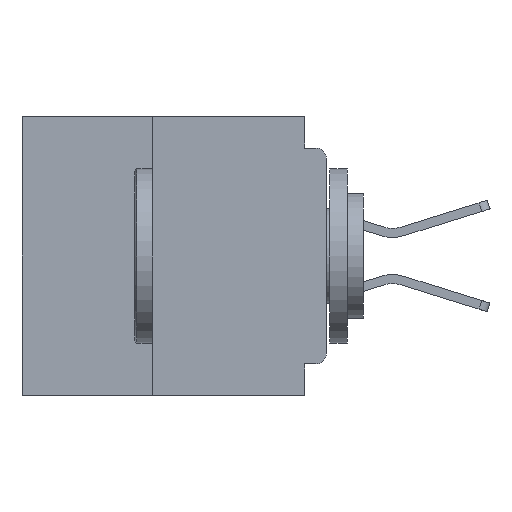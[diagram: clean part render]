
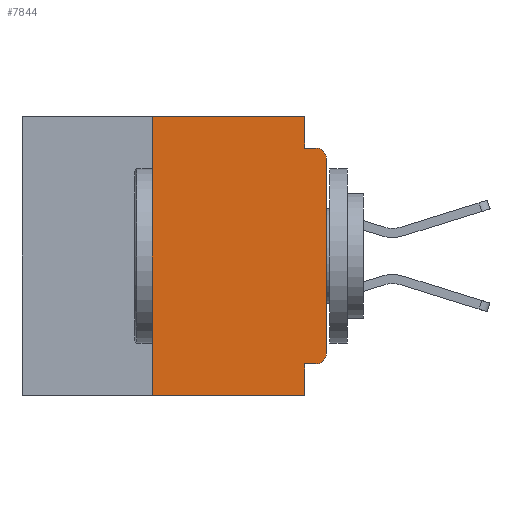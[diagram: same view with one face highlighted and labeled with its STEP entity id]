
A CAD part, left-side view. The second image highlights one B-rep face of the part: STEP entity #7844.
In plain terms, the highlighted planar face has unit normal (-1, 0, 0).
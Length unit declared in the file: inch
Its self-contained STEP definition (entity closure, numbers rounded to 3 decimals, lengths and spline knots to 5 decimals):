
#17 = EDGE_CURVE ( 'NONE', #37100, #36242, #29036, .T. ) ;
#1278 = DIRECTION ( 'NONE',  ( -1., 0., 0. ) ) ;
#3343 = CARTESIAN_POINT ( 'NONE',  ( 0., 0., -0.34 ) ) ;
#3614 = CARTESIAN_POINT ( 'NONE',  ( 0., 0.031, 0. ) ) ;
#3674 = LINE ( 'NONE', #17124, #46001 ) ;
#4310 = DIRECTION ( 'NONE',  ( -1., 0., 0. ) ) ;
#5064 = VECTOR ( 'NONE', #15952, 39.37008 ) ;
#5339 = CARTESIAN_POINT ( 'NONE',  ( 0., 0.25, -0.4 ) ) ;
#6149 = VERTEX_POINT ( 'NONE', #40076 ) ;
#6697 = PLANE ( 'NONE',  #9297 ) ;
#6918 = VECTOR ( 'NONE', #46391, 39.37008 ) ;
#7844 = ADVANCED_FACE ( 'NONE', ( #22489 ), #6697, .F. ) ;
#8098 = CIRCLE ( 'NONE', #25250, 0.015 ) ;
#9297 = AXIS2_PLACEMENT_3D ( 'NONE', #43621, #19162, #47717 ) ;
#9511 = LINE ( 'NONE', #15062, #20519 ) ;
#9533 = EDGE_CURVE ( 'NONE', #40594, #33171, #8098, .T. ) ;
#11437 = EDGE_CURVE ( 'NONE', #38877, #35262, #44872, .T. ) ;
#13422 = DIRECTION ( 'NONE',  ( 0., -1., 0. ) ) ;
#13489 = CARTESIAN_POINT ( 'NONE',  ( 0., 0.25, -0.4 ) ) ;
#13791 = VERTEX_POINT ( 'NONE', #50449 ) ;
#15062 = CARTESIAN_POINT ( 'NONE',  ( 0., 0., -0.355 ) ) ;
#15172 = VERTEX_POINT ( 'NONE', #24614 ) ;
#15555 = ORIENTED_EDGE ( 'NONE', *, *, #27257, .F. ) ;
#15952 = DIRECTION ( 'NONE',  ( 0., -1., 0. ) ) ;
#15962 = DIRECTION ( 'NONE',  ( 0., -1., 0. ) ) ;
#17124 = CARTESIAN_POINT ( 'NONE',  ( 0., 0.031, -0.4 ) ) ;
#17565 = CARTESIAN_POINT ( 'NONE',  ( 0., 0.437, -0.4 ) ) ;
#18684 = ORIENTED_EDGE ( 'NONE', *, *, #9533, .T. ) ;
#19162 = DIRECTION ( 'NONE',  ( 1., 0., 0. ) ) ;
#19197 = DIRECTION ( 'NONE',  ( 0., 1., 0. ) ) ;
#20519 = VECTOR ( 'NONE', #19197, 39.37008 ) ;
#21345 = AXIS2_PLACEMENT_3D ( 'NONE', #29032, #4310, #33144 ) ;
#21432 = CARTESIAN_POINT ( 'NONE',  ( 0., 0.015, -0.355 ) ) ;
#21860 = EDGE_CURVE ( 'NONE', #40594, #6149, #9511, .T. ) ;
#21900 = LINE ( 'NONE', #48632, #23185 ) ;
#22489 = FACE_OUTER_BOUND ( 'NONE', #43771, .T. ) ;
#23185 = VECTOR ( 'NONE', #15962, 39.37008 ) ;
#24335 = DIRECTION ( 'NONE',  ( 0., 0., -1. ) ) ;
#24614 = CARTESIAN_POINT ( 'NONE',  ( 0., 0., -0.06 ) ) ;
#25250 = AXIS2_PLACEMENT_3D ( 'NONE', #26008, #1278, #30164 ) ;
#26008 = CARTESIAN_POINT ( 'NONE',  ( 0., 0.015, -0.34 ) ) ;
#26440 = ORIENTED_EDGE ( 'NONE', *, *, #46007, .F. ) ;
#27059 = ORIENTED_EDGE ( 'NONE', *, *, #40671, .F. ) ;
#27257 = EDGE_CURVE ( 'NONE', #36242, #51646, #21900, .T. ) ;
#28770 = ORIENTED_EDGE ( 'NONE', *, *, #11437, .T. ) ;
#29032 = CARTESIAN_POINT ( 'NONE',  ( 0., 0.015, -0.06 ) ) ;
#29036 = LINE ( 'NONE', #3614, #49361 ) ;
#29613 = EDGE_CURVE ( 'NONE', #15172, #51646, #49452, .T. ) ;
#29731 = DIRECTION ( 'NONE',  ( 0., 0., -1. ) ) ;
#30164 = DIRECTION ( 'NONE',  ( 0., 0., -1. ) ) ;
#30694 = CARTESIAN_POINT ( 'NONE',  ( 0., 0.015, -0.045 ) ) ;
#30896 = CARTESIAN_POINT ( 'NONE',  ( 0., 0.031, -0.4 ) ) ;
#30962 = ORIENTED_EDGE ( 'NONE', *, *, #21860, .F. ) ;
#30990 = VECTOR ( 'NONE', #48415, 39.37008 ) ;
#31171 = ORIENTED_EDGE ( 'NONE', *, *, #32830, .F. ) ;
#32254 = LINE ( 'NONE', #52461, #30990 ) ;
#32830 = EDGE_CURVE ( 'NONE', #6149, #35262, #3674, .T. ) ;
#33144 = DIRECTION ( 'NONE',  ( 0., 0., -1. ) ) ;
#33171 = VERTEX_POINT ( 'NONE', #3343 ) ;
#35262 = VERTEX_POINT ( 'NONE', #30896 ) ;
#35463 = EDGE_CURVE ( 'NONE', #33171, #15172, #32254, .T. ) ;
#36242 = VERTEX_POINT ( 'NONE', #37512 ) ;
#37100 = VERTEX_POINT ( 'NONE', #47719 ) ;
#37512 = CARTESIAN_POINT ( 'NONE',  ( 0., 0.031, -0.045 ) ) ;
#38877 = VERTEX_POINT ( 'NONE', #13489 ) ;
#39149 = LINE ( 'NONE', #48460, #5064 ) ;
#39688 = LINE ( 'NONE', #5339, #6918 ) ;
#40076 = CARTESIAN_POINT ( 'NONE',  ( 0., 0.031, -0.355 ) ) ;
#40594 = VERTEX_POINT ( 'NONE', #21432 ) ;
#40671 = EDGE_CURVE ( 'NONE', #38877, #13791, #39688, .T. ) ;
#41267 = ORIENTED_EDGE ( 'NONE', *, *, #29613, .T. ) ;
#41938 = ORIENTED_EDGE ( 'NONE', *, *, #17, .F. ) ;
#43565 = VECTOR ( 'NONE', #13422, 39.37008 ) ;
#43621 = CARTESIAN_POINT ( 'NONE',  ( 0., 0.437, 0. ) ) ;
#43771 = EDGE_LOOP ( 'NONE', ( #46137, #41267, #15555, #41938, #26440, #27059, #28770, #31171, #30962, #18684 ) ) ;
#44872 = LINE ( 'NONE', #17565, #43565 ) ;
#46001 = VECTOR ( 'NONE', #29731, 39.37008 ) ;
#46007 = EDGE_CURVE ( 'NONE', #13791, #37100, #39149, .T. ) ;
#46137 = ORIENTED_EDGE ( 'NONE', *, *, #35463, .T. ) ;
#46391 = DIRECTION ( 'NONE',  ( 0., 0., 1. ) ) ;
#47717 = DIRECTION ( 'NONE',  ( 0., 0., -1. ) ) ;
#47719 = CARTESIAN_POINT ( 'NONE',  ( 0., 0.031, 0. ) ) ;
#48415 = DIRECTION ( 'NONE',  ( 0., 0., 1. ) ) ;
#48460 = CARTESIAN_POINT ( 'NONE',  ( 0., 0.437, 0. ) ) ;
#48632 = CARTESIAN_POINT ( 'NONE',  ( 0., 0., -0.045 ) ) ;
#49361 = VECTOR ( 'NONE', #24335, 39.37008 ) ;
#49452 = CIRCLE ( 'NONE', #21345, 0.015 ) ;
#50449 = CARTESIAN_POINT ( 'NONE',  ( 0., 0.25, 0. ) ) ;
#51646 = VERTEX_POINT ( 'NONE', #30694 ) ;
#52461 = CARTESIAN_POINT ( 'NONE',  ( 0., 0., 0. ) ) ;
